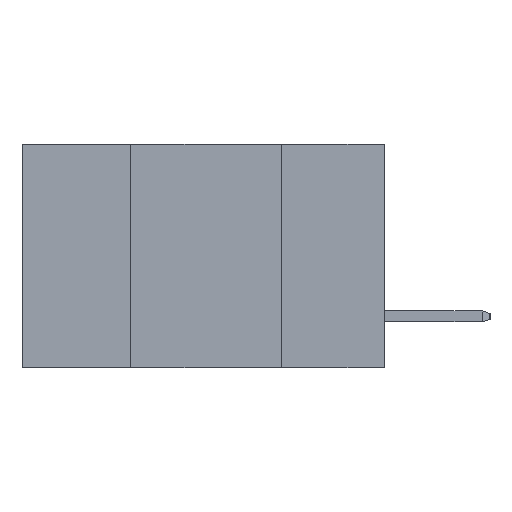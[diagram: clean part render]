
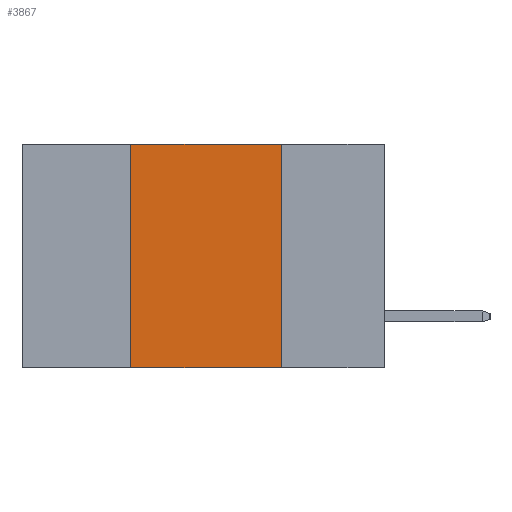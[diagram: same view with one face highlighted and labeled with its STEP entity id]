
A CAD part, left-side view. The second image highlights one B-rep face of the part: STEP entity #3867.
In plain terms, the highlighted planar face has unit normal (-1, 0, 0).
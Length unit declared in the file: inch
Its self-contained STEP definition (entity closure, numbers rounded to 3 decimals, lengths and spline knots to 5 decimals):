
#339 = CARTESIAN_POINT ( 'NONE',  ( 0., 0.17, 0. ) ) ;
#886 = VECTOR ( 'NONE', #5361, 39.37008 ) ;
#1788 = LINE ( 'NONE', #5806, #886 ) ;
#1866 = EDGE_LOOP ( 'NONE', ( #10143, #3585, #8124, #2982 ) ) ;
#2102 = VERTEX_POINT ( 'NONE', #5734 ) ;
#2752 = DIRECTION ( 'NONE',  ( 0., 0., -1. ) ) ;
#2868 = DIRECTION ( 'NONE',  ( 1., 0., 0. ) ) ;
#2918 = CARTESIAN_POINT ( 'NONE',  ( 0., 0.6, 0. ) ) ;
#2982 = ORIENTED_EDGE ( 'NONE', *, *, #5230, .T. ) ;
#3035 = PLANE ( 'NONE',  #11425 ) ;
#3219 = CARTESIAN_POINT ( 'NONE',  ( 0., 0.6, 0. ) ) ;
#3408 = LINE ( 'NONE', #8081, #7677 ) ;
#3577 = DIRECTION ( 'NONE',  ( 0., -1., 0. ) ) ;
#3585 = ORIENTED_EDGE ( 'NONE', *, *, #6346, .F. ) ;
#3867 = ADVANCED_FACE ( 'NONE', ( #4998 ), #3035, .F. ) ;
#4366 = VERTEX_POINT ( 'NONE', #5424 ) ;
#4445 = LINE ( 'NONE', #4943, #8401 ) ;
#4943 = CARTESIAN_POINT ( 'NONE',  ( 0., 0.6, -0.37 ) ) ;
#4998 = FACE_OUTER_BOUND ( 'NONE', #1866, .T. ) ;
#5055 = DIRECTION ( 'NONE',  ( 0., -1., 0. ) ) ;
#5230 = EDGE_CURVE ( 'NONE', #7368, #4366, #4445, .T. ) ;
#5361 = DIRECTION ( 'NONE',  ( 0., 0., 1. ) ) ;
#5424 = CARTESIAN_POINT ( 'NONE',  ( 0., 0.17, -0.37 ) ) ;
#5476 = DIRECTION ( 'NONE',  ( 0., 0., -1. ) ) ;
#5734 = CARTESIAN_POINT ( 'NONE',  ( 0., 0.42, 0. ) ) ;
#5779 = EDGE_CURVE ( 'NONE', #7368, #2102, #1788, .T. ) ;
#5806 = CARTESIAN_POINT ( 'NONE',  ( 0., 0.42, -0.37 ) ) ;
#6346 = EDGE_CURVE ( 'NONE', #2102, #8829, #8366, .T. ) ;
#6883 = CARTESIAN_POINT ( 'NONE',  ( 0., 0.42, -0.37 ) ) ;
#6914 = EDGE_CURVE ( 'NONE', #8829, #4366, #3408, .T. ) ;
#7368 = VERTEX_POINT ( 'NONE', #6883 ) ;
#7677 = VECTOR ( 'NONE', #5476, 39.37008 ) ;
#8081 = CARTESIAN_POINT ( 'NONE',  ( 0., 0.17, -0.37 ) ) ;
#8124 = ORIENTED_EDGE ( 'NONE', *, *, #5779, .F. ) ;
#8366 = LINE ( 'NONE', #3219, #10924 ) ;
#8401 = VECTOR ( 'NONE', #5055, 39.37008 ) ;
#8829 = VERTEX_POINT ( 'NONE', #339 ) ;
#10143 = ORIENTED_EDGE ( 'NONE', *, *, #6914, .F. ) ;
#10924 = VECTOR ( 'NONE', #3577, 39.37008 ) ;
#11425 = AXIS2_PLACEMENT_3D ( 'NONE', #2918, #2868, #2752 ) ;
